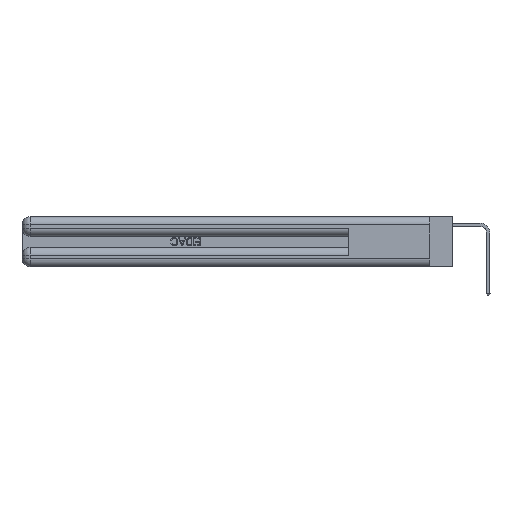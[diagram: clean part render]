
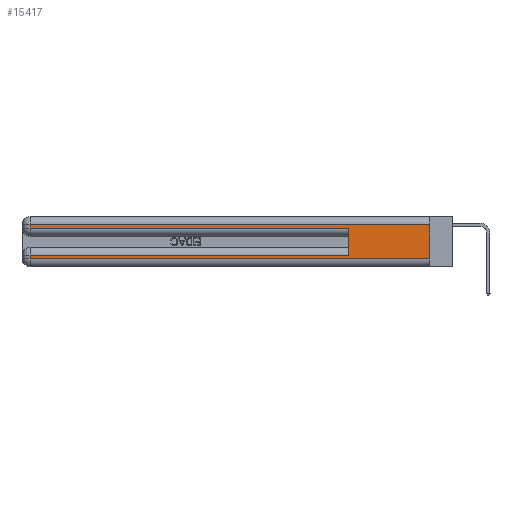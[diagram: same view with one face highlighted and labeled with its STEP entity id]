
A CAD part, left-side view. The second image highlights one B-rep face of the part: STEP entity #15417.
In plain terms, the highlighted planar face has unit normal (-1, 0, 0).
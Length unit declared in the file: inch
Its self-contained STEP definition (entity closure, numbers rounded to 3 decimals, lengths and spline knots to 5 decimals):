
#470 = VECTOR ( 'NONE', #4549, 39.37008 ) ;
#1789 = VERTEX_POINT ( 'NONE', #5762 ) ;
#2091 = DIRECTION ( 'NONE',  ( 0., 1., 0. ) ) ;
#2477 = CARTESIAN_POINT ( 'NONE',  ( 0., 2.94, 0.37 ) ) ;
#3117 = CARTESIAN_POINT ( 'NONE',  ( 0., 2.94, 0.085 ) ) ;
#4339 = EDGE_CURVE ( 'NONE', #28087, #21592, #32637, .T. ) ;
#4549 = DIRECTION ( 'NONE',  ( 0., 0., -1. ) ) ;
#4893 = CARTESIAN_POINT ( 'NONE',  ( 0., 0.6, 0.145 ) ) ;
#4904 = VERTEX_POINT ( 'NONE', #25442 ) ;
#5762 = CARTESIAN_POINT ( 'NONE',  ( 0., 2.94, 0.06 ) ) ;
#6701 = EDGE_CURVE ( 'NONE', #19361, #30957, #18153, .T. ) ;
#6714 = EDGE_CURVE ( 'NONE', #4904, #19361, #27637, .T. ) ;
#6871 = DIRECTION ( 'NONE',  ( 0., 0., -1. ) ) ;
#7044 = FACE_OUTER_BOUND ( 'NONE', #26934, .T. ) ;
#7393 = ORIENTED_EDGE ( 'NONE', *, *, #4339, .F. ) ;
#7413 = CARTESIAN_POINT ( 'NONE',  ( 0., 2.94, 0.285 ) ) ;
#7414 = AXIS2_PLACEMENT_3D ( 'NONE', #21744, #8918, #6871 ) ;
#7417 = DIRECTION ( 'NONE',  ( 0., -1., 0. ) ) ;
#8601 = CARTESIAN_POINT ( 'NONE',  ( 0., 0.6, 0.085 ) ) ;
#8918 = DIRECTION ( 'NONE',  ( 1., 0., 0. ) ) ;
#9767 = VECTOR ( 'NONE', #17756, 39.37008 ) ;
#10614 = VECTOR ( 'NONE', #2091, 39.37008 ) ;
#10767 = VERTEX_POINT ( 'NONE', #3117 ) ;
#11709 = DIRECTION ( 'NONE',  ( 0., 1., 0. ) ) ;
#11902 = CARTESIAN_POINT ( 'NONE',  ( 0., 0., 0.085 ) ) ;
#14351 = EDGE_CURVE ( 'NONE', #28865, #10767, #27717, .T. ) ;
#15206 = VECTOR ( 'NONE', #30039, 39.37008 ) ;
#15370 = ORIENTED_EDGE ( 'NONE', *, *, #24726, .T. ) ;
#15417 = ADVANCED_FACE ( 'NONE', ( #7044 ), #24426, .F. ) ;
#16320 = ORIENTED_EDGE ( 'NONE', *, *, #27571, .F. ) ;
#17241 = CARTESIAN_POINT ( 'NONE',  ( 0., 0., 0.31 ) ) ;
#17723 = LINE ( 'NONE', #27838, #15206 ) ;
#17756 = DIRECTION ( 'NONE',  ( 0., 0., -1. ) ) ;
#18153 = LINE ( 'NONE', #28417, #26324 ) ;
#18883 = EDGE_CURVE ( 'NONE', #10767, #1789, #17723, .T. ) ;
#19361 = VERTEX_POINT ( 'NONE', #7413 ) ;
#19435 = LINE ( 'NONE', #17241, #23260 ) ;
#21592 = VERTEX_POINT ( 'NONE', #31346 ) ;
#21744 = CARTESIAN_POINT ( 'NONE',  ( 0., 0., 0.37 ) ) ;
#22207 = VECTOR ( 'NONE', #7417, 39.37008 ) ;
#22288 = VECTOR ( 'NONE', #28318, 39.37008 ) ;
#22327 = CARTESIAN_POINT ( 'NONE',  ( 0., 0., 0.31 ) ) ;
#22331 = ORIENTED_EDGE ( 'NONE', *, *, #23823, .T. ) ;
#22776 = LINE ( 'NONE', #4893, #22288 ) ;
#22836 = CARTESIAN_POINT ( 'NONE',  ( 0., 0., 0.37 ) ) ;
#23260 = VECTOR ( 'NONE', #11709, 39.37008 ) ;
#23823 = EDGE_CURVE ( 'NONE', #28087, #4904, #19435, .T. ) ;
#24426 = PLANE ( 'NONE',  #7414 ) ;
#24726 = EDGE_CURVE ( 'NONE', #1789, #21592, #25957, .T. ) ;
#24802 = ORIENTED_EDGE ( 'NONE', *, *, #14351, .T. ) ;
#25442 = CARTESIAN_POINT ( 'NONE',  ( 0., 2.94, 0.31 ) ) ;
#25957 = LINE ( 'NONE', #26127, #22207 ) ;
#26127 = CARTESIAN_POINT ( 'NONE',  ( 0., 0., 0.06 ) ) ;
#26324 = VECTOR ( 'NONE', #32731, 39.37008 ) ;
#26934 = EDGE_LOOP ( 'NONE', ( #7393, #22331, #31542, #30643, #16320, #24802, #32349, #15370 ) ) ;
#27571 = EDGE_CURVE ( 'NONE', #28865, #30957, #22776, .T. ) ;
#27637 = LINE ( 'NONE', #2477, #470 ) ;
#27717 = LINE ( 'NONE', #11902, #10614 ) ;
#27838 = CARTESIAN_POINT ( 'NONE',  ( 0., 2.94, 0.37 ) ) ;
#28087 = VERTEX_POINT ( 'NONE', #22327 ) ;
#28318 = DIRECTION ( 'NONE',  ( 0., 0., 1. ) ) ;
#28406 = CARTESIAN_POINT ( 'NONE',  ( 0., 0.6, 0.285 ) ) ;
#28417 = CARTESIAN_POINT ( 'NONE',  ( 0., 0., 0.285 ) ) ;
#28865 = VERTEX_POINT ( 'NONE', #8601 ) ;
#30039 = DIRECTION ( 'NONE',  ( 0., 0., -1. ) ) ;
#30643 = ORIENTED_EDGE ( 'NONE', *, *, #6701, .T. ) ;
#30957 = VERTEX_POINT ( 'NONE', #28406 ) ;
#31346 = CARTESIAN_POINT ( 'NONE',  ( 0., 0., 0.06 ) ) ;
#31542 = ORIENTED_EDGE ( 'NONE', *, *, #6714, .T. ) ;
#32349 = ORIENTED_EDGE ( 'NONE', *, *, #18883, .T. ) ;
#32637 = LINE ( 'NONE', #22836, #9767 ) ;
#32731 = DIRECTION ( 'NONE',  ( 0., -1., 0. ) ) ;
